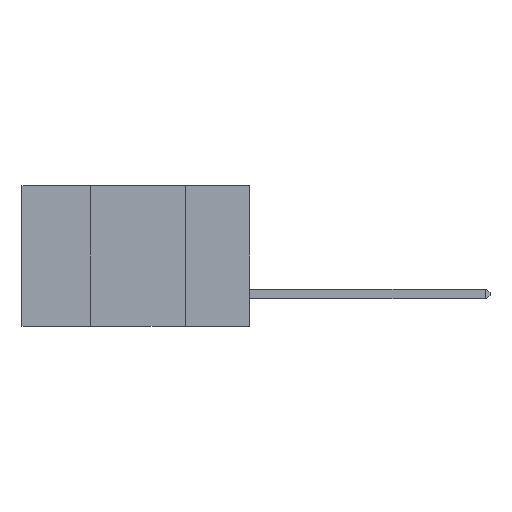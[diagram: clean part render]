
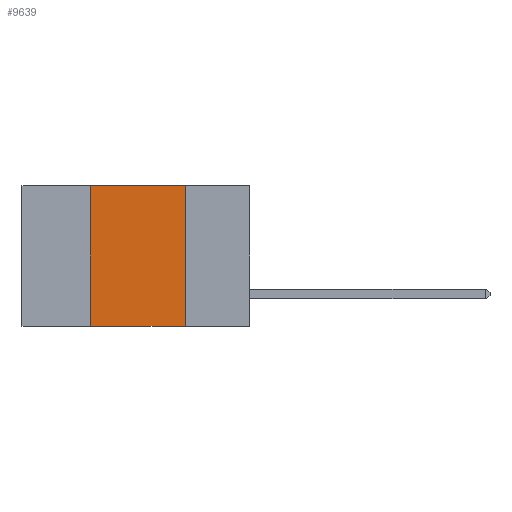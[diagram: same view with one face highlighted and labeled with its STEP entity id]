
A CAD part, left-side view. The second image highlights one B-rep face of the part: STEP entity #9639.
In plain terms, the highlighted planar face has unit normal (-1, 0, 0).
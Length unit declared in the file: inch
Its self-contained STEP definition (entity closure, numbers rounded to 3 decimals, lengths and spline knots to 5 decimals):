
#339 = VERTEX_POINT ( 'NONE', #8314 ) ;
#788 = CARTESIAN_POINT ( 'NONE',  ( 0., 0.17, 0. ) ) ;
#1007 = VECTOR ( 'NONE', #1783, 39.37008 ) ;
#1024 = AXIS2_PLACEMENT_3D ( 'NONE', #9141, #4296, #9861 ) ;
#1516 = CARTESIAN_POINT ( 'NONE',  ( 0., 0.17, -0.37 ) ) ;
#1783 = DIRECTION ( 'NONE',  ( 0., 0., -1. ) ) ;
#2159 = CARTESIAN_POINT ( 'NONE',  ( 0., 0.42, -0.37 ) ) ;
#2458 = CARTESIAN_POINT ( 'NONE',  ( 0., 0.6, -0.37 ) ) ;
#2748 = EDGE_CURVE ( 'NONE', #339, #7712, #10540, .T. ) ;
#3435 = ORIENTED_EDGE ( 'NONE', *, *, #2748, .F. ) ;
#3448 = ORIENTED_EDGE ( 'NONE', *, *, #6664, .F. ) ;
#3674 = DIRECTION ( 'NONE',  ( 0., -1., 0. ) ) ;
#3694 = VERTEX_POINT ( 'NONE', #1516 ) ;
#3713 = ORIENTED_EDGE ( 'NONE', *, *, #9006, .F. ) ;
#3793 = ORIENTED_EDGE ( 'NONE', *, *, #7169, .T. ) ;
#3934 = LINE ( 'NONE', #2458, #5939 ) ;
#4250 = DIRECTION ( 'NONE',  ( 0., 0., 1. ) ) ;
#4296 = DIRECTION ( 'NONE',  ( 1., 0., 0. ) ) ;
#4593 = CARTESIAN_POINT ( 'NONE',  ( 0., 0.6, 0. ) ) ;
#5939 = VECTOR ( 'NONE', #9030, 39.37008 ) ;
#6664 = EDGE_CURVE ( 'NONE', #7712, #3694, #9814, .T. ) ;
#7037 = LINE ( 'NONE', #8355, #8871 ) ;
#7169 = EDGE_CURVE ( 'NONE', #7446, #3694, #3934, .T. ) ;
#7446 = VERTEX_POINT ( 'NONE', #2159 ) ;
#7711 = FACE_OUTER_BOUND ( 'NONE', #8820, .T. ) ;
#7712 = VERTEX_POINT ( 'NONE', #8305 ) ;
#8305 = CARTESIAN_POINT ( 'NONE',  ( 0., 0.17, 0. ) ) ;
#8314 = CARTESIAN_POINT ( 'NONE',  ( 0., 0.42, 0. ) ) ;
#8355 = CARTESIAN_POINT ( 'NONE',  ( 0., 0.42, 0. ) ) ;
#8404 = PLANE ( 'NONE',  #1024 ) ;
#8635 = VECTOR ( 'NONE', #3674, 39.37008 ) ;
#8820 = EDGE_LOOP ( 'NONE', ( #3448, #3435, #3713, #3793 ) ) ;
#8871 = VECTOR ( 'NONE', #4250, 39.37008 ) ;
#9006 = EDGE_CURVE ( 'NONE', #7446, #339, #7037, .T. ) ;
#9030 = DIRECTION ( 'NONE',  ( 0., -1., 0. ) ) ;
#9141 = CARTESIAN_POINT ( 'NONE',  ( 0., 0.6, 0. ) ) ;
#9639 = ADVANCED_FACE ( 'NONE', ( #7711 ), #8404, .F. ) ;
#9814 = LINE ( 'NONE', #788, #1007 ) ;
#9861 = DIRECTION ( 'NONE',  ( 0., 0., -1. ) ) ;
#10540 = LINE ( 'NONE', #4593, #8635 ) ;
